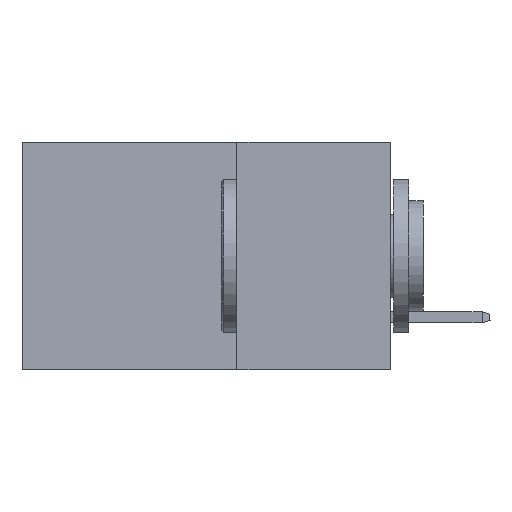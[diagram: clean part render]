
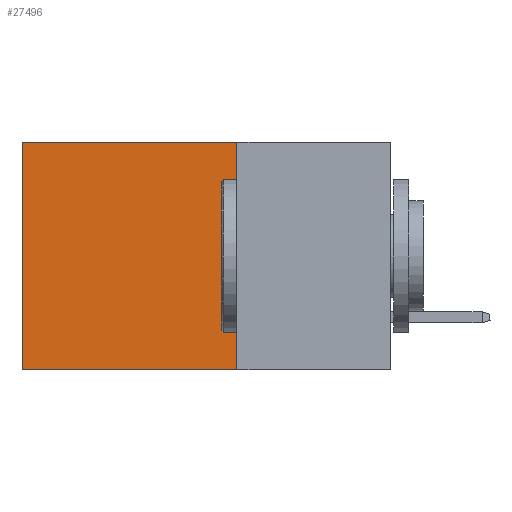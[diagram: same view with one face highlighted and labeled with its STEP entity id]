
A CAD part, left-side view. The second image highlights one B-rep face of the part: STEP entity #27496.
In plain terms, the highlighted planar face has unit normal (-1, 0, 0).
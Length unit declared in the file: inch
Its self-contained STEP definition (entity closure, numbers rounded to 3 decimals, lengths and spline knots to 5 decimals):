
#208 = ORIENTED_EDGE ( 'NONE', *, *, #31334, .T. ) ;
#403 = AXIS2_PLACEMENT_3D ( 'NONE', #29408, #8613, #6075 ) ;
#5609 = ORIENTED_EDGE ( 'NONE', *, *, #33259, .F. ) ;
#5793 = CARTESIAN_POINT ( 'NONE',  ( 0.2875, 0.6, 0. ) ) ;
#5843 = PLANE ( 'NONE',  #403 ) ;
#6075 = DIRECTION ( 'NONE',  ( 0., 0., -1. ) ) ;
#6284 = VECTOR ( 'NONE', #17341, 39.37008 ) ;
#6486 = LINE ( 'NONE', #21729, #22632 ) ;
#7227 = VERTEX_POINT ( 'NONE', #12197 ) ;
#7418 = EDGE_LOOP ( 'NONE', ( #208, #14354, #5609, #24899 ) ) ;
#8613 = DIRECTION ( 'NONE',  ( 1., 0., 0. ) ) ;
#10900 = VERTEX_POINT ( 'NONE', #21004 ) ;
#12197 = CARTESIAN_POINT ( 'NONE',  ( 0.2875, 0.25, 0. ) ) ;
#13544 = FACE_OUTER_BOUND ( 'NONE', #7418, .T. ) ;
#13744 = EDGE_CURVE ( 'NONE', #7227, #16343, #6486, .T. ) ;
#14354 = ORIENTED_EDGE ( 'NONE', *, *, #27911, .F. ) ;
#15639 = VECTOR ( 'NONE', #29388, 39.37008 ) ;
#16343 = VERTEX_POINT ( 'NONE', #5793 ) ;
#17341 = DIRECTION ( 'NONE',  ( 0., 0., -1. ) ) ;
#20172 = LINE ( 'NONE', #24066, #15639 ) ;
#21004 = CARTESIAN_POINT ( 'NONE',  ( 0.2875, 0.25, -0.37 ) ) ;
#21503 = DIRECTION ( 'NONE',  ( 0., 1., 0. ) ) ;
#21696 = CARTESIAN_POINT ( 'NONE',  ( 0.2875, 0.6, 0. ) ) ;
#21729 = CARTESIAN_POINT ( 'NONE',  ( 0.2875, 0.25, 0. ) ) ;
#22376 = CARTESIAN_POINT ( 'NONE',  ( 0.2875, 0.25, 0. ) ) ;
#22632 = VECTOR ( 'NONE', #21503, 39.37008 ) ;
#23520 = VECTOR ( 'NONE', #33371, 39.37008 ) ;
#24066 = CARTESIAN_POINT ( 'NONE',  ( 0.2875, 0.25, -0.37 ) ) ;
#24326 = LINE ( 'NONE', #22376, #23520 ) ;
#24899 = ORIENTED_EDGE ( 'NONE', *, *, #13744, .T. ) ;
#27152 = VERTEX_POINT ( 'NONE', #31360 ) ;
#27496 = ADVANCED_FACE ( 'NONE', ( #13544 ), #5843, .F. ) ;
#27911 = EDGE_CURVE ( 'NONE', #10900, #27152, #20172, .T. ) ;
#29388 = DIRECTION ( 'NONE',  ( 0., 1., 0. ) ) ;
#29408 = CARTESIAN_POINT ( 'NONE',  ( 0.2875, 0.25, 0. ) ) ;
#31334 = EDGE_CURVE ( 'NONE', #16343, #27152, #31515, .T. ) ;
#31360 = CARTESIAN_POINT ( 'NONE',  ( 0.2875, 0.6, -0.37 ) ) ;
#31515 = LINE ( 'NONE', #21696, #6284 ) ;
#33259 = EDGE_CURVE ( 'NONE', #7227, #10900, #24326, .T. ) ;
#33371 = DIRECTION ( 'NONE',  ( 0., 0., -1. ) ) ;
